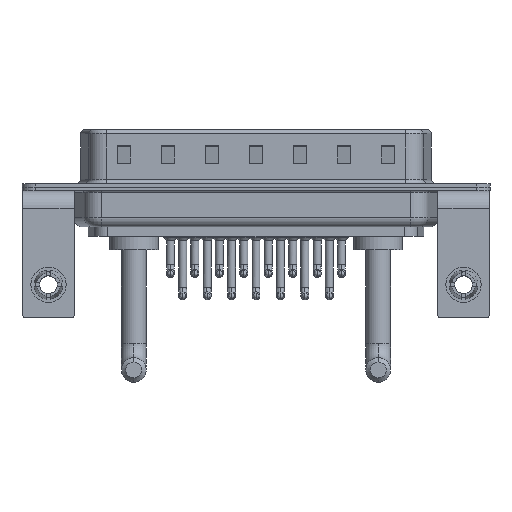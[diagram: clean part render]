
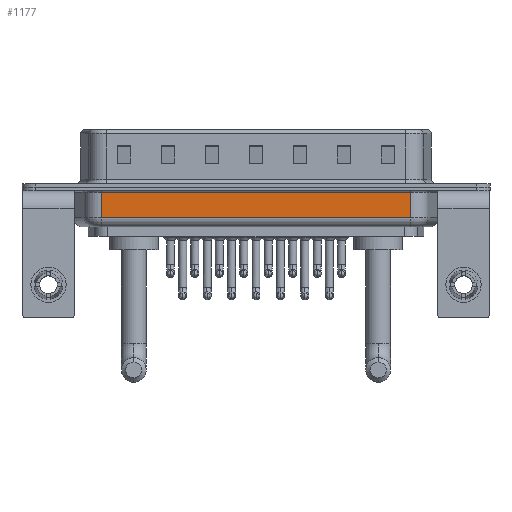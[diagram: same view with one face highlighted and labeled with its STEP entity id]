
A CAD part, front view. The second image highlights one B-rep face of the part: STEP entity #1177.
In plain terms, the highlighted planar face has unit normal (0, -1, 0).
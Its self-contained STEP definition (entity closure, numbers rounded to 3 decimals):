
#349 = VECTOR ( 'NONE', #7635, 1000. ) ;
#607 = VECTOR ( 'NONE', #11688, 1000. ) ;
#1009 = LINE ( 'NONE', #17748, #22859 ) ;
#1083 = EDGE_CURVE ( 'NONE', #6681, #14412, #12095, .T. ) ;
#1177 = ADVANCED_FACE ( 'NONE', ( #15657 ), #5231, .F. ) ;
#1179 = ORIENTED_EDGE ( 'NONE', *, *, #23038, .F. ) ;
#3186 = DIRECTION ( 'NONE',  ( 0., 0., 1. ) ) ;
#3547 = ORIENTED_EDGE ( 'NONE', *, *, #15201, .T. ) ;
#3589 = CARTESIAN_POINT ( 'NONE',  ( 6.006, -5.35, -3.5 ) ) ;
#3601 = CARTESIAN_POINT ( 'NONE',  ( 41.044, -5.35, -3.5 ) ) ;
#3907 = LINE ( 'NONE', #8039, #349 ) ;
#5231 = PLANE ( 'NONE',  #23442 ) ;
#6681 = VERTEX_POINT ( 'NONE', #12868 ) ;
#7635 = DIRECTION ( 'NONE',  ( -1., 0., 0. ) ) ;
#7935 = VERTEX_POINT ( 'NONE', #22578 ) ;
#8039 = CARTESIAN_POINT ( 'NONE',  ( 6.006, -5.35, -0.65 ) ) ;
#9769 = ORIENTED_EDGE ( 'NONE', *, *, #21275, .T. ) ;
#11447 = CARTESIAN_POINT ( 'NONE',  ( 6.006, -5.35, -4.5 ) ) ;
#11688 = DIRECTION ( 'NONE',  ( 1., 0., 0. ) ) ;
#12095 = LINE ( 'NONE', #3589, #607 ) ;
#12868 = CARTESIAN_POINT ( 'NONE',  ( 6.006, -5.35, -3.5 ) ) ;
#13033 = ORIENTED_EDGE ( 'NONE', *, *, #1083, .T. ) ;
#13613 = CARTESIAN_POINT ( 'NONE',  ( 6.006, -5.35, -4.5 ) ) ;
#13945 = CARTESIAN_POINT ( 'NONE',  ( 41.044, -5.35, -0.65 ) ) ;
#14412 = VERTEX_POINT ( 'NONE', #3601 ) ;
#15201 = EDGE_CURVE ( 'NONE', #14412, #16096, #1009, .T. ) ;
#15657 = FACE_OUTER_BOUND ( 'NONE', #17781, .T. ) ;
#16096 = VERTEX_POINT ( 'NONE', #13945 ) ;
#17748 = CARTESIAN_POINT ( 'NONE',  ( 41.044, -5.35, -4.5 ) ) ;
#17781 = EDGE_LOOP ( 'NONE', ( #1179, #13033, #3547, #9769 ) ) ;
#17888 = DIRECTION ( 'NONE',  ( 0., 0., 1. ) ) ;
#20614 = VECTOR ( 'NONE', #17888, 1000. ) ;
#21275 = EDGE_CURVE ( 'NONE', #16096, #7935, #3907, .T. ) ;
#21988 = DIRECTION ( 'NONE',  ( 0., 1., 0. ) ) ;
#22578 = CARTESIAN_POINT ( 'NONE',  ( 6.006, -5.35, -0.65 ) ) ;
#22859 = VECTOR ( 'NONE', #26374, 1000. ) ;
#23038 = EDGE_CURVE ( 'NONE', #6681, #7935, #23522, .T. ) ;
#23442 = AXIS2_PLACEMENT_3D ( 'NONE', #13613, #21988, #3186 ) ;
#23522 = LINE ( 'NONE', #11447, #20614 ) ;
#26374 = DIRECTION ( 'NONE',  ( 0., 0., 1. ) ) ;
